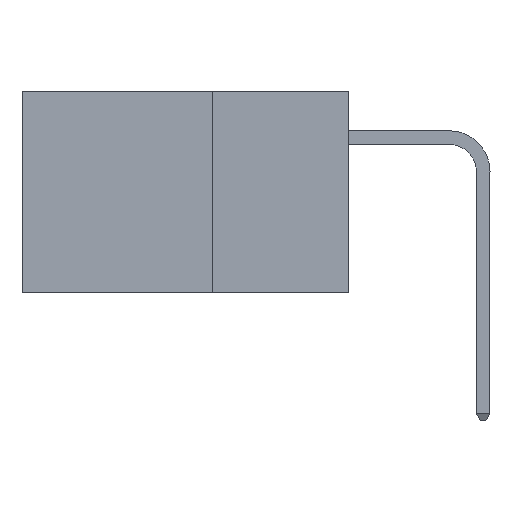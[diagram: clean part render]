
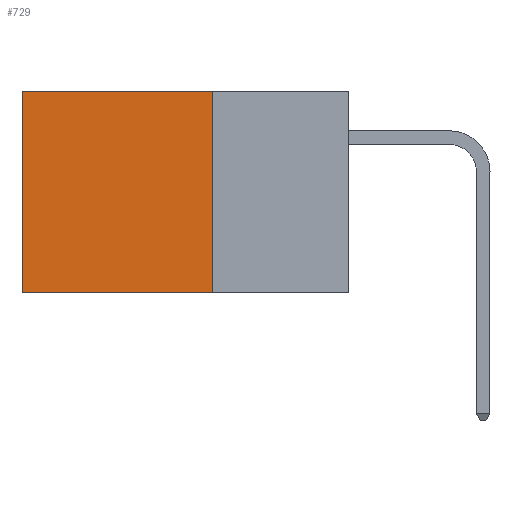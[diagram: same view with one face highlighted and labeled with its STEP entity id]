
A CAD part, left-side view. The second image highlights one B-rep face of the part: STEP entity #729.
In plain terms, the highlighted planar face has unit normal (-1, 0, 0).
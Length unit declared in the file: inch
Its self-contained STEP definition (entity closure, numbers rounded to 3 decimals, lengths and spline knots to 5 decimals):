
#91 = EDGE_CURVE ( 'NONE', #4793, #1352, #11466, .T. ) ;
#112 = PLANE ( 'NONE',  #11301 ) ;
#295 = ORIENTED_EDGE ( 'NONE', *, *, #2986, .T. ) ;
#729 = ADVANCED_FACE ( 'NONE', ( #20245 ), #112, .F. ) ;
#981 = EDGE_CURVE ( 'NONE', #1352, #6333, #22465, .T. ) ;
#1185 = EDGE_CURVE ( 'NONE', #4793, #10259, #21894, .T. ) ;
#1352 = VERTEX_POINT ( 'NONE', #17838 ) ;
#2986 = EDGE_CURVE ( 'NONE', #10259, #6333, #15589, .T. ) ;
#4507 = DIRECTION ( 'NONE',  ( 0., 0., -1. ) ) ;
#4737 = VECTOR ( 'NONE', #16312, 39.37008 ) ;
#4793 = VERTEX_POINT ( 'NONE', #13506 ) ;
#4826 = EDGE_LOOP ( 'NONE', ( #295, #18110, #7258, #11558 ) ) ;
#5206 = CARTESIAN_POINT ( 'NONE',  ( 0.2875, 0.25, 0. ) ) ;
#5359 = DIRECTION ( 'NONE',  ( 0., 0., -1. ) ) ;
#6333 = VERTEX_POINT ( 'NONE', #19374 ) ;
#7258 = ORIENTED_EDGE ( 'NONE', *, *, #91, .F. ) ;
#7703 = CARTESIAN_POINT ( 'NONE',  ( 0.2875, 0.25, 0. ) ) ;
#8657 = VECTOR ( 'NONE', #19640, 39.37008 ) ;
#9165 = CARTESIAN_POINT ( 'NONE',  ( 0.2875, 0.25, -0.37 ) ) ;
#10259 = VERTEX_POINT ( 'NONE', #18348 ) ;
#10869 = VECTOR ( 'NONE', #4507, 39.37008 ) ;
#11301 = AXIS2_PLACEMENT_3D ( 'NONE', #5206, #17624, #5359 ) ;
#11466 = LINE ( 'NONE', #14340, #8657 ) ;
#11526 = DIRECTION ( 'NONE',  ( 0., 1., 0. ) ) ;
#11558 = ORIENTED_EDGE ( 'NONE', *, *, #1185, .T. ) ;
#13506 = CARTESIAN_POINT ( 'NONE',  ( 0.2875, 0.25, 0. ) ) ;
#14340 = CARTESIAN_POINT ( 'NONE',  ( 0.2875, 0.25, 0. ) ) ;
#15228 = CARTESIAN_POINT ( 'NONE',  ( 0.2875, 0.6, 0. ) ) ;
#15589 = LINE ( 'NONE', #15228, #10869 ) ;
#16312 = DIRECTION ( 'NONE',  ( 0., 1., 0. ) ) ;
#17213 = VECTOR ( 'NONE', #11526, 39.37008 ) ;
#17624 = DIRECTION ( 'NONE',  ( 1., 0., 0. ) ) ;
#17838 = CARTESIAN_POINT ( 'NONE',  ( 0.2875, 0.25, -0.37 ) ) ;
#18110 = ORIENTED_EDGE ( 'NONE', *, *, #981, .F. ) ;
#18348 = CARTESIAN_POINT ( 'NONE',  ( 0.2875, 0.6, 0. ) ) ;
#19374 = CARTESIAN_POINT ( 'NONE',  ( 0.2875, 0.6, -0.37 ) ) ;
#19640 = DIRECTION ( 'NONE',  ( 0., 0., -1. ) ) ;
#20245 = FACE_OUTER_BOUND ( 'NONE', #4826, .T. ) ;
#21894 = LINE ( 'NONE', #7703, #17213 ) ;
#22465 = LINE ( 'NONE', #9165, #4737 ) ;
